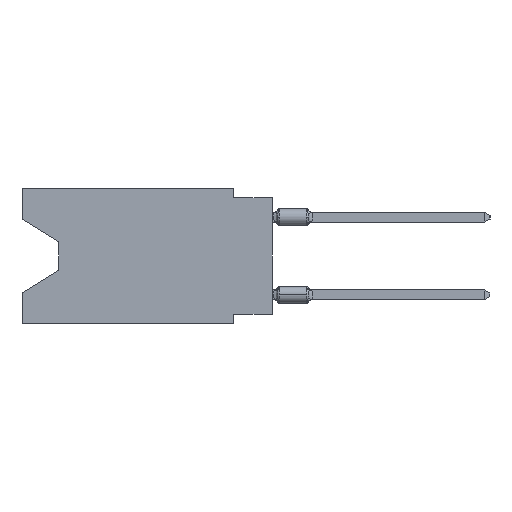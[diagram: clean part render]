
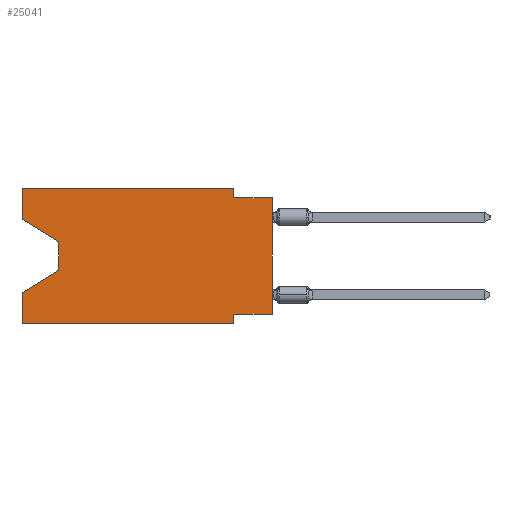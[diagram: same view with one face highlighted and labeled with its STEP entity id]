
A CAD part, left-side view. The second image highlights one B-rep face of the part: STEP entity #25041.
In plain terms, the highlighted planar face has unit normal (-1, 0, 0).
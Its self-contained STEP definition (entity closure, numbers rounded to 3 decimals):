
#920 = DIRECTION ( 'NONE',  ( 1., 0., 0. ) ) ;
#1235 = CARTESIAN_POINT ( 'NONE',  ( 0., 16.383, 0. ) ) ;
#1551 = DIRECTION ( 'NONE',  ( 0., 0., 1. ) ) ;
#2291 = EDGE_CURVE ( 'NONE', #6627, #37435, #17044, .T. ) ;
#2615 = LINE ( 'NONE', #41930, #40427 ) ;
#2838 = DIRECTION ( 'NONE',  ( 0., 0., 1. ) ) ;
#3253 = VECTOR ( 'NONE', #5962, 1000. ) ;
#3376 = DIRECTION ( 'NONE',  ( 0., 0., 1. ) ) ;
#3812 = CARTESIAN_POINT ( 'NONE',  ( 0., 13.97, -3.505 ) ) ;
#3978 = AXIS2_PLACEMENT_3D ( 'NONE', #18915, #920, #15348 ) ;
#4245 = PLANE ( 'NONE',  #3978 ) ;
#4478 = FACE_OUTER_BOUND ( 'NONE', #31626, .T. ) ;
#4862 = VERTEX_POINT ( 'NONE', #8666 ) ;
#5107 = CARTESIAN_POINT ( 'NONE',  ( 0., 0., 0. ) ) ;
#5962 = DIRECTION ( 'NONE',  ( 0., -1., 0. ) ) ;
#6058 = CARTESIAN_POINT ( 'NONE',  ( 0., 0., -0.635 ) ) ;
#6156 = CARTESIAN_POINT ( 'NONE',  ( 0., 16.383, -8.89 ) ) ;
#6627 = VERTEX_POINT ( 'NONE', #6156 ) ;
#6915 = LINE ( 'NONE', #21355, #34236 ) ;
#7119 = DIRECTION ( 'NONE',  ( 0., 0., -1. ) ) ;
#7317 = EDGE_CURVE ( 'NONE', #36083, #11501, #36245, .T. ) ;
#7767 = CARTESIAN_POINT ( 'NONE',  ( 0., 2.54, 0. ) ) ;
#8666 = CARTESIAN_POINT ( 'NONE',  ( 0., 2.54, -8.89 ) ) ;
#9212 = ORIENTED_EDGE ( 'NONE', *, *, #17759, .F. ) ;
#10362 = EDGE_CURVE ( 'NONE', #44423, #32400, #39281, .T. ) ;
#11210 = ORIENTED_EDGE ( 'NONE', *, *, #40338, .F. ) ;
#11501 = VERTEX_POINT ( 'NONE', #25632 ) ;
#13284 = CARTESIAN_POINT ( 'NONE',  ( 0., 0., -0.635 ) ) ;
#14380 = DIRECTION ( 'NONE',  ( 0., 0., -1. ) ) ;
#14700 = VERTEX_POINT ( 'NONE', #45209 ) ;
#15348 = DIRECTION ( 'NONE',  ( 0., 0., -1. ) ) ;
#15353 = VECTOR ( 'NONE', #22220, 1000. ) ;
#16461 = CARTESIAN_POINT ( 'NONE',  ( 0., 16.383, 0. ) ) ;
#17023 = ORIENTED_EDGE ( 'NONE', *, *, #32211, .T. ) ;
#17044 = LINE ( 'NONE', #35033, #31548 ) ;
#17704 = CARTESIAN_POINT ( 'NONE',  ( 0., 13.97, -3.505 ) ) ;
#17759 = EDGE_CURVE ( 'NONE', #44987, #42493, #33791, .T. ) ;
#18915 = CARTESIAN_POINT ( 'NONE',  ( 0., 16.383, 0. ) ) ;
#19769 = CARTESIAN_POINT ( 'NONE',  ( 0., 16.383, -2.038 ) ) ;
#19989 = EDGE_CURVE ( 'NONE', #6627, #4862, #21788, .T. ) ;
#21151 = CARTESIAN_POINT ( 'NONE',  ( 0., 0., -8.255 ) ) ;
#21355 = CARTESIAN_POINT ( 'NONE',  ( 0., 16.383, 0. ) ) ;
#21788 = LINE ( 'NONE', #36226, #39419 ) ;
#21810 = ORIENTED_EDGE ( 'NONE', *, *, #35398, .T. ) ;
#22220 = DIRECTION ( 'NONE',  ( 0., 0., -1. ) ) ;
#23360 = CARTESIAN_POINT ( 'NONE',  ( 0., 2.54, 0. ) ) ;
#25041 = ADVANCED_FACE ( 'NONE', ( #4478 ), #4245, .F. ) ;
#25240 = ORIENTED_EDGE ( 'NONE', *, *, #7317, .T. ) ;
#25632 = CARTESIAN_POINT ( 'NONE',  ( 0., 13.97, -5.385 ) ) ;
#26715 = CARTESIAN_POINT ( 'NONE',  ( 0., 2.54, -0.635 ) ) ;
#26877 = VERTEX_POINT ( 'NONE', #1235 ) ;
#27021 = LINE ( 'NONE', #13284, #3253 ) ;
#27527 = ORIENTED_EDGE ( 'NONE', *, *, #19989, .T. ) ;
#28850 = EDGE_CURVE ( 'NONE', #14700, #36083, #37288, .T. ) ;
#29057 = CARTESIAN_POINT ( 'NONE',  ( 0., 2.54, -8.89 ) ) ;
#30910 = DIRECTION ( 'NONE',  ( 0., -1., 0. ) ) ;
#31267 = VECTOR ( 'NONE', #1551, 1000. ) ;
#31354 = EDGE_CURVE ( 'NONE', #26877, #44423, #34696, .T. ) ;
#31362 = VERTEX_POINT ( 'NONE', #6058 ) ;
#31548 = VECTOR ( 'NONE', #2838, 1000. ) ;
#31626 = EDGE_LOOP ( 'NONE', ( #38132, #25240, #17023, #39635, #27527, #38332, #9212, #21810, #33450, #33876, #38640, #11210 ) ) ;
#32211 = EDGE_CURVE ( 'NONE', #11501, #37435, #2615, .T. ) ;
#32400 = VERTEX_POINT ( 'NONE', #26715 ) ;
#32840 = LINE ( 'NONE', #29057, #38607 ) ;
#33450 = ORIENTED_EDGE ( 'NONE', *, *, #39062, .F. ) ;
#33680 = VECTOR ( 'NONE', #34203, 1000. ) ;
#33791 = LINE ( 'NONE', #37804, #35456 ) ;
#33876 = ORIENTED_EDGE ( 'NONE', *, *, #10362, .F. ) ;
#34203 = DIRECTION ( 'NONE',  ( 0., -0.855, -0.519 ) ) ;
#34236 = VECTOR ( 'NONE', #3376, 1000. ) ;
#34317 = VECTOR ( 'NONE', #30910, 1000. ) ;
#34696 = LINE ( 'NONE', #16461, #34317 ) ;
#34820 = DIRECTION ( 'NONE',  ( 0., 0.855, -0.519 ) ) ;
#35033 = CARTESIAN_POINT ( 'NONE',  ( 0., 16.383, 0. ) ) ;
#35398 = EDGE_CURVE ( 'NONE', #44987, #31362, #44870, .T. ) ;
#35456 = VECTOR ( 'NONE', #37572, 1000. ) ;
#36083 = VERTEX_POINT ( 'NONE', #17704 ) ;
#36226 = CARTESIAN_POINT ( 'NONE',  ( 0., 16.383, -8.89 ) ) ;
#36245 = LINE ( 'NONE', #3812, #45874 ) ;
#36452 = DIRECTION ( 'NONE',  ( 0., -1., 0. ) ) ;
#36664 = EDGE_CURVE ( 'NONE', #42493, #4862, #32840, .T. ) ;
#37288 = LINE ( 'NONE', #19769, #33680 ) ;
#37435 = VERTEX_POINT ( 'NONE', #38434 ) ;
#37572 = DIRECTION ( 'NONE',  ( 0., 1., 0. ) ) ;
#37804 = CARTESIAN_POINT ( 'NONE',  ( 0., 0., -8.255 ) ) ;
#38132 = ORIENTED_EDGE ( 'NONE', *, *, #28850, .T. ) ;
#38332 = ORIENTED_EDGE ( 'NONE', *, *, #36664, .F. ) ;
#38434 = CARTESIAN_POINT ( 'NONE',  ( 0., 16.383, -6.852 ) ) ;
#38607 = VECTOR ( 'NONE', #14380, 1000. ) ;
#38640 = ORIENTED_EDGE ( 'NONE', *, *, #31354, .F. ) ;
#39062 = EDGE_CURVE ( 'NONE', #32400, #31362, #27021, .T. ) ;
#39281 = LINE ( 'NONE', #7767, #15353 ) ;
#39348 = CARTESIAN_POINT ( 'NONE',  ( 0., 2.54, -8.255 ) ) ;
#39419 = VECTOR ( 'NONE', #36452, 1000. ) ;
#39635 = ORIENTED_EDGE ( 'NONE', *, *, #2291, .F. ) ;
#40338 = EDGE_CURVE ( 'NONE', #14700, #26877, #6915, .T. ) ;
#40427 = VECTOR ( 'NONE', #34820, 1000. ) ;
#41930 = CARTESIAN_POINT ( 'NONE',  ( 0., 13.97, -5.385 ) ) ;
#42493 = VERTEX_POINT ( 'NONE', #39348 ) ;
#44423 = VERTEX_POINT ( 'NONE', #23360 ) ;
#44870 = LINE ( 'NONE', #5107, #31267 ) ;
#44987 = VERTEX_POINT ( 'NONE', #21151 ) ;
#45209 = CARTESIAN_POINT ( 'NONE',  ( 0., 16.383, -2.038 ) ) ;
#45874 = VECTOR ( 'NONE', #7119, 1000. ) ;
